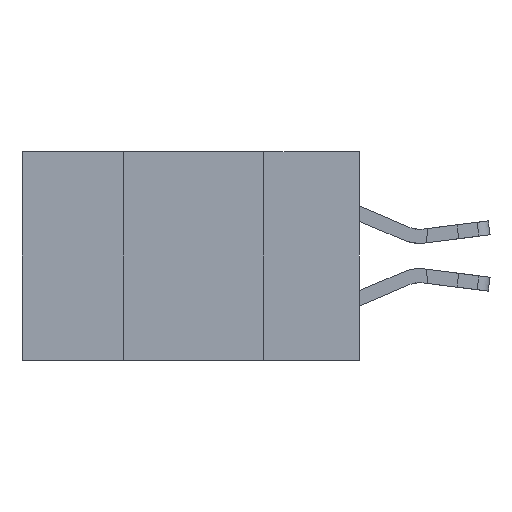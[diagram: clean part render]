
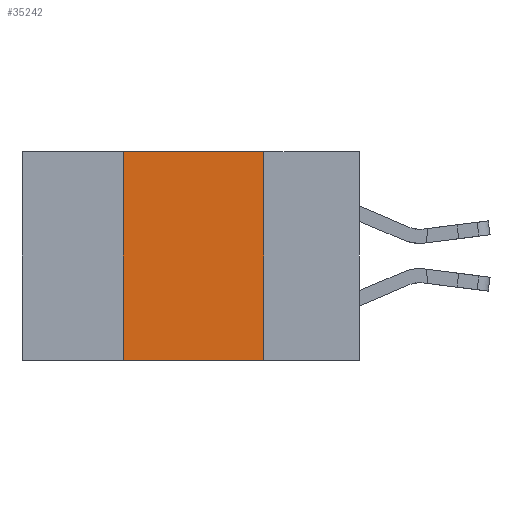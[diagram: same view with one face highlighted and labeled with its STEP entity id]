
A CAD part, left-side view. The second image highlights one B-rep face of the part: STEP entity #35242.
In plain terms, the highlighted planar face has unit normal (-1, 0, 0).
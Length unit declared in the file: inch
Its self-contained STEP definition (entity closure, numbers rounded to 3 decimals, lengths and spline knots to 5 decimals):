
#199 = LINE ( 'NONE', #26744, #28317 ) ;
#1536 = EDGE_CURVE ( 'NONE', #5122, #29433, #25434, .T. ) ;
#1551 = CARTESIAN_POINT ( 'NONE',  ( 0., 0.6, -0.37 ) ) ;
#1918 = DIRECTION ( 'NONE',  ( 0., -1., 0. ) ) ;
#2018 = DIRECTION ( 'NONE',  ( 0., 0., -1. ) ) ;
#4003 = VECTOR ( 'NONE', #7067, 39.37008 ) ;
#4566 = CARTESIAN_POINT ( 'NONE',  ( 0., 0.6, 0. ) ) ;
#5122 = VERTEX_POINT ( 'NONE', #11347 ) ;
#7067 = DIRECTION ( 'NONE',  ( 0., -1., 0. ) ) ;
#8121 = ORIENTED_EDGE ( 'NONE', *, *, #24602, .T. ) ;
#9349 = EDGE_CURVE ( 'NONE', #25601, #34808, #199, .T. ) ;
#10226 = CARTESIAN_POINT ( 'NONE',  ( 0., 0.42, 0. ) ) ;
#11335 = DIRECTION ( 'NONE',  ( 0., 0., -1. ) ) ;
#11347 = CARTESIAN_POINT ( 'NONE',  ( 0., 0.42, -0.37 ) ) ;
#11509 = VECTOR ( 'NONE', #1918, 39.37008 ) ;
#14956 = ORIENTED_EDGE ( 'NONE', *, *, #1536, .F. ) ;
#17098 = ORIENTED_EDGE ( 'NONE', *, *, #20152, .F. ) ;
#20152 = EDGE_CURVE ( 'NONE', #29433, #25601, #22737, .T. ) ;
#22146 = DIRECTION ( 'NONE',  ( 1., 0., 0. ) ) ;
#22633 = CARTESIAN_POINT ( 'NONE',  ( 0., 0.17, -0.37 ) ) ;
#22737 = LINE ( 'NONE', #4566, #4003 ) ;
#24277 = LINE ( 'NONE', #1551, #11509 ) ;
#24602 = EDGE_CURVE ( 'NONE', #5122, #34808, #24277, .T. ) ;
#25337 = CARTESIAN_POINT ( 'NONE',  ( 0., 0.6, 0. ) ) ;
#25369 = EDGE_LOOP ( 'NONE', ( #29040, #17098, #14956, #8121 ) ) ;
#25434 = LINE ( 'NONE', #10226, #28424 ) ;
#25601 = VERTEX_POINT ( 'NONE', #32902 ) ;
#26179 = AXIS2_PLACEMENT_3D ( 'NONE', #25337, #22146, #11335 ) ;
#26744 = CARTESIAN_POINT ( 'NONE',  ( 0., 0.17, 0. ) ) ;
#27852 = DIRECTION ( 'NONE',  ( 0., 0., 1. ) ) ;
#27951 = PLANE ( 'NONE',  #26179 ) ;
#28317 = VECTOR ( 'NONE', #2018, 39.37008 ) ;
#28424 = VECTOR ( 'NONE', #27852, 39.37008 ) ;
#29040 = ORIENTED_EDGE ( 'NONE', *, *, #9349, .F. ) ;
#29433 = VERTEX_POINT ( 'NONE', #33345 ) ;
#32902 = CARTESIAN_POINT ( 'NONE',  ( 0., 0.17, 0. ) ) ;
#33345 = CARTESIAN_POINT ( 'NONE',  ( 0., 0.42, 0. ) ) ;
#33516 = FACE_OUTER_BOUND ( 'NONE', #25369, .T. ) ;
#34808 = VERTEX_POINT ( 'NONE', #22633 ) ;
#35242 = ADVANCED_FACE ( 'NONE', ( #33516 ), #27951, .F. ) ;
